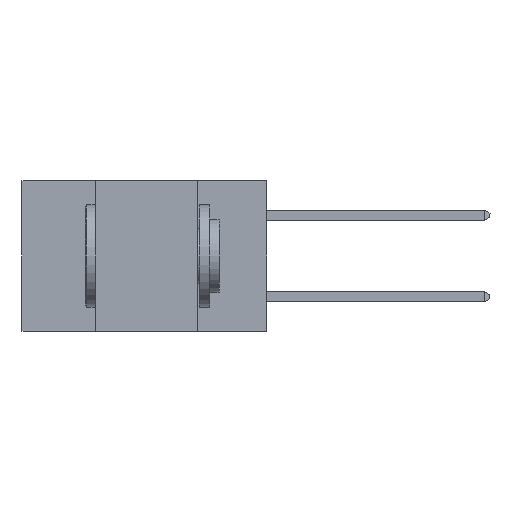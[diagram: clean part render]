
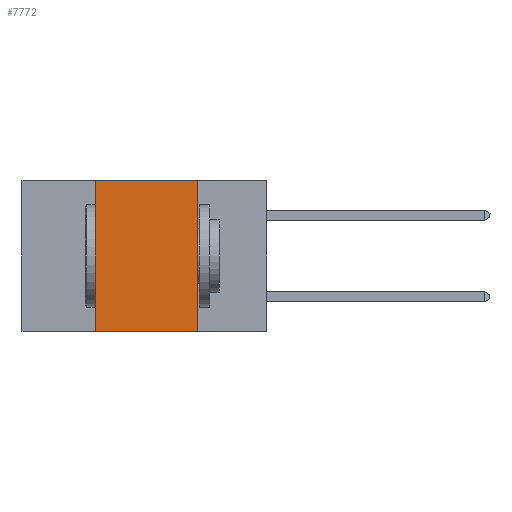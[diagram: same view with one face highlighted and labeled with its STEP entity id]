
A CAD part, left-side view. The second image highlights one B-rep face of the part: STEP entity #7772.
In plain terms, the highlighted planar face has unit normal (-1, 0, 0).
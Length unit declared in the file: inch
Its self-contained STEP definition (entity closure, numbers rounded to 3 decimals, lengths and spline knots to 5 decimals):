
#275 = DIRECTION ( 'NONE',  ( 0., 0., -1. ) ) ;
#400 = VECTOR ( 'NONE', #5624, 39.37008 ) ;
#481 = VERTEX_POINT ( 'NONE', #2105 ) ;
#748 = LINE ( 'NONE', #4530, #400 ) ;
#854 = CARTESIAN_POINT ( 'NONE',  ( 0., 0.17, 0. ) ) ;
#907 = DIRECTION ( 'NONE',  ( 0., 0., -1. ) ) ;
#984 = LINE ( 'NONE', #854, #6483 ) ;
#1044 = CARTESIAN_POINT ( 'NONE',  ( 0., 0.17, 0. ) ) ;
#1221 = EDGE_LOOP ( 'NONE', ( #11949, #6873, #12251, #1389 ) ) ;
#1389 = ORIENTED_EDGE ( 'NONE', *, *, #1853, .T. ) ;
#1422 = AXIS2_PLACEMENT_3D ( 'NONE', #11910, #6850, #275 ) ;
#1853 = EDGE_CURVE ( 'NONE', #10908, #11768, #2066, .T. ) ;
#2066 = LINE ( 'NONE', #13044, #5330 ) ;
#2105 = CARTESIAN_POINT ( 'NONE',  ( 0., 0.42, 0. ) ) ;
#4349 = VERTEX_POINT ( 'NONE', #1044 ) ;
#4530 = CARTESIAN_POINT ( 'NONE',  ( 0., 0.6, 0. ) ) ;
#4671 = PLANE ( 'NONE',  #1422 ) ;
#4716 = VECTOR ( 'NONE', #7311, 39.37008 ) ;
#5330 = VECTOR ( 'NONE', #12921, 39.37008 ) ;
#5337 = EDGE_CURVE ( 'NONE', #4349, #11768, #984, .T. ) ;
#5624 = DIRECTION ( 'NONE',  ( 0., -1., 0. ) ) ;
#6483 = VECTOR ( 'NONE', #907, 39.37008 ) ;
#6850 = DIRECTION ( 'NONE',  ( 1., 0., 0. ) ) ;
#6873 = ORIENTED_EDGE ( 'NONE', *, *, #7654, .F. ) ;
#7045 = CARTESIAN_POINT ( 'NONE',  ( 0., 0.17, -0.37 ) ) ;
#7311 = DIRECTION ( 'NONE',  ( 0., 0., 1. ) ) ;
#7654 = EDGE_CURVE ( 'NONE', #481, #4349, #748, .T. ) ;
#7772 = ADVANCED_FACE ( 'NONE', ( #10454 ), #4671, .F. ) ;
#7970 = EDGE_CURVE ( 'NONE', #10908, #481, #12904, .T. ) ;
#9344 = CARTESIAN_POINT ( 'NONE',  ( 0., 0.42, 0. ) ) ;
#9758 = CARTESIAN_POINT ( 'NONE',  ( 0., 0.42, -0.37 ) ) ;
#10454 = FACE_OUTER_BOUND ( 'NONE', #1221, .T. ) ;
#10908 = VERTEX_POINT ( 'NONE', #9758 ) ;
#11768 = VERTEX_POINT ( 'NONE', #7045 ) ;
#11910 = CARTESIAN_POINT ( 'NONE',  ( 0., 0.6, 0. ) ) ;
#11949 = ORIENTED_EDGE ( 'NONE', *, *, #5337, .F. ) ;
#12251 = ORIENTED_EDGE ( 'NONE', *, *, #7970, .F. ) ;
#12904 = LINE ( 'NONE', #9344, #4716 ) ;
#12921 = DIRECTION ( 'NONE',  ( 0., -1., 0. ) ) ;
#13044 = CARTESIAN_POINT ( 'NONE',  ( 0., 0.6, -0.37 ) ) ;
